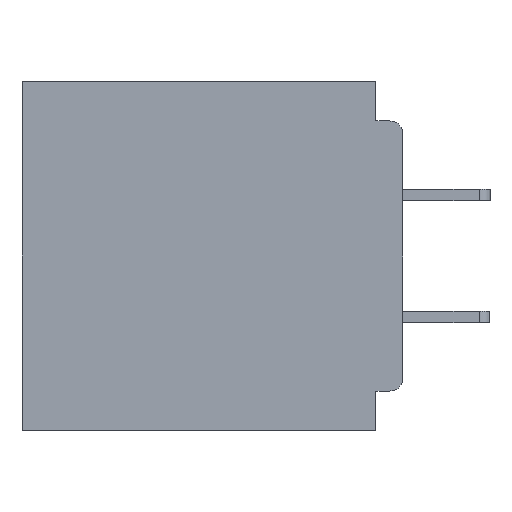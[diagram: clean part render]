
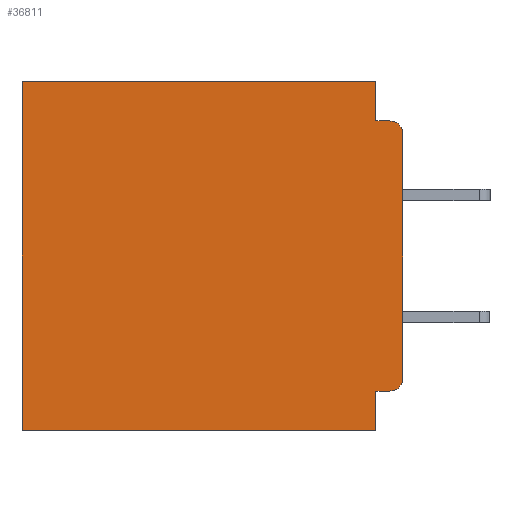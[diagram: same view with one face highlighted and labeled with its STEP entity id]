
A CAD part, left-side view. The second image highlights one B-rep face of the part: STEP entity #36811.
In plain terms, the highlighted planar face has unit normal (-1, 0, 0).
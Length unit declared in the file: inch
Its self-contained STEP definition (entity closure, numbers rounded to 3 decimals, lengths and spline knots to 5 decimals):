
#180 = LINE ( 'NONE', #29104, #8390 ) ;
#1345 = VERTEX_POINT ( 'NONE', #10909 ) ;
#2168 = DIRECTION ( 'NONE',  ( -1., 0., 0. ) ) ;
#2389 = CARTESIAN_POINT ( 'NONE',  ( 0.3, 0., -0.355 ) ) ;
#2405 = CARTESIAN_POINT ( 'NONE',  ( 0.3, 0., -0.34 ) ) ;
#3158 = CARTESIAN_POINT ( 'NONE',  ( 0.3, 0., -0.4 ) ) ;
#3338 = LINE ( 'NONE', #4510, #16851 ) ;
#3372 = CARTESIAN_POINT ( 'NONE',  ( 0.3, 0.015, -0.06 ) ) ;
#4238 = LINE ( 'NONE', #2389, #20634 ) ;
#4364 = VECTOR ( 'NONE', #32236, 39.37008 ) ;
#4455 = AXIS2_PLACEMENT_3D ( 'NONE', #7632, #10760, #32193 ) ;
#4510 = CARTESIAN_POINT ( 'NONE',  ( 0.3, 0., 0. ) ) ;
#4531 = PLANE ( 'NONE',  #4455 ) ;
#4718 = VERTEX_POINT ( 'NONE', #17786 ) ;
#5389 = CARTESIAN_POINT ( 'NONE',  ( 0.3, 0.031, -0.045 ) ) ;
#5960 = VERTEX_POINT ( 'NONE', #30890 ) ;
#6119 = VECTOR ( 'NONE', #23405, 39.37008 ) ;
#6398 = CARTESIAN_POINT ( 'NONE',  ( 0.3, 0.031, -0.355 ) ) ;
#6465 = DIRECTION ( 'NONE',  ( 0., 0., -1. ) ) ;
#7095 = LINE ( 'NONE', #20351, #6119 ) ;
#7237 = VECTOR ( 'NONE', #30842, 39.37008 ) ;
#7554 = VERTEX_POINT ( 'NONE', #36003 ) ;
#7614 = DIRECTION ( 'NONE',  ( 0., 1., 0. ) ) ;
#7632 = CARTESIAN_POINT ( 'NONE',  ( 0.3, 0., -0.4 ) ) ;
#7782 = EDGE_LOOP ( 'NONE', ( #23162, #24529, #25824, #27682, #28188, #29527, #30024, #30924, #31496, #32269 ) ) ;
#7936 = LINE ( 'NONE', #35241, #31489 ) ;
#8390 = VECTOR ( 'NONE', #16808, 39.37008 ) ;
#8595 = EDGE_CURVE ( 'NONE', #29781, #26532, #3338, .T. ) ;
#10760 = DIRECTION ( 'NONE',  ( 1., 0., 0. ) ) ;
#10909 = CARTESIAN_POINT ( 'NONE',  ( 0.3, 0.015, -0.045 ) ) ;
#13442 = EDGE_CURVE ( 'NONE', #5960, #7554, #7936, .T. ) ;
#13830 = CARTESIAN_POINT ( 'NONE',  ( 0.3, 0.437, 0. ) ) ;
#13949 = LINE ( 'NONE', #29820, #29267 ) ;
#14097 = VERTEX_POINT ( 'NONE', #5389 ) ;
#14298 = EDGE_CURVE ( 'NONE', #4718, #1345, #24211, .T. ) ;
#16808 = DIRECTION ( 'NONE',  ( 0., -1., 0. ) ) ;
#16851 = VECTOR ( 'NONE', #7614, 39.37008 ) ;
#16928 = DIRECTION ( 'NONE',  ( 0., 1., 0. ) ) ;
#17786 = CARTESIAN_POINT ( 'NONE',  ( 0.3, 0., -0.06 ) ) ;
#17795 = DIRECTION ( 'NONE',  ( 0., 1., 0. ) ) ;
#19812 = EDGE_CURVE ( 'NONE', #20315, #37203, #4238, .T. ) ;
#20315 = VERTEX_POINT ( 'NONE', #38423 ) ;
#20351 = CARTESIAN_POINT ( 'NONE',  ( 0.3, 0.031, 0. ) ) ;
#20634 = VECTOR ( 'NONE', #17795, 39.37008 ) ;
#20643 = CARTESIAN_POINT ( 'NONE',  ( 0.3, 0.015, -0.34 ) ) ;
#21900 = EDGE_CURVE ( 'NONE', #14097, #1345, #180, .T. ) ;
#23162 = ORIENTED_EDGE ( 'NONE', *, *, #24052, .F. ) ;
#23405 = DIRECTION ( 'NONE',  ( 0., 0., -1. ) ) ;
#23693 = DIRECTION ( 'NONE',  ( 0., 0., -1. ) ) ;
#24052 = EDGE_CURVE ( 'NONE', #4718, #35542, #31728, .T. ) ;
#24075 = CARTESIAN_POINT ( 'NONE',  ( 0.3, 0.031, 0. ) ) ;
#24211 = CIRCLE ( 'NONE', #37267, 0.015 ) ;
#24529 = ORIENTED_EDGE ( 'NONE', *, *, #14298, .T. ) ;
#24862 = DIRECTION ( 'NONE',  ( -1., 0., 0. ) ) ;
#25824 = ORIENTED_EDGE ( 'NONE', *, *, #21900, .F. ) ;
#26532 = VERTEX_POINT ( 'NONE', #13830 ) ;
#27682 = ORIENTED_EDGE ( 'NONE', *, *, #38051, .F. ) ;
#27984 = CIRCLE ( 'NONE', #35754, 0.015 ) ;
#28188 = ORIENTED_EDGE ( 'NONE', *, *, #8595, .T. ) ;
#29033 = CARTESIAN_POINT ( 'NONE',  ( 0.3, 0.031, -0.4 ) ) ;
#29104 = CARTESIAN_POINT ( 'NONE',  ( 0.3, 0., -0.045 ) ) ;
#29267 = VECTOR ( 'NONE', #35996, 39.37008 ) ;
#29527 = ORIENTED_EDGE ( 'NONE', *, *, #36347, .T. ) ;
#29781 = VERTEX_POINT ( 'NONE', #24075 ) ;
#29820 = CARTESIAN_POINT ( 'NONE',  ( 0.3, 0.437, -0.4 ) ) ;
#30024 = ORIENTED_EDGE ( 'NONE', *, *, #13442, .F. ) ;
#30842 = DIRECTION ( 'NONE',  ( 0., 0., -1. ) ) ;
#30890 = CARTESIAN_POINT ( 'NONE',  ( 0.3, 0.031, -0.4 ) ) ;
#30924 = ORIENTED_EDGE ( 'NONE', *, *, #35329, .F. ) ;
#31489 = VECTOR ( 'NONE', #16928, 39.37008 ) ;
#31496 = ORIENTED_EDGE ( 'NONE', *, *, #19812, .F. ) ;
#31728 = LINE ( 'NONE', #3158, #7237 ) ;
#32193 = DIRECTION ( 'NONE',  ( 0., 0., -1. ) ) ;
#32236 = DIRECTION ( 'NONE',  ( 0., 0., -1. ) ) ;
#32269 = ORIENTED_EDGE ( 'NONE', *, *, #33003, .T. ) ;
#33003 = EDGE_CURVE ( 'NONE', #20315, #35542, #27984, .T. ) ;
#35241 = CARTESIAN_POINT ( 'NONE',  ( 0.3, 0., -0.4 ) ) ;
#35329 = EDGE_CURVE ( 'NONE', #37203, #5960, #36079, .T. ) ;
#35542 = VERTEX_POINT ( 'NONE', #2405 ) ;
#35754 = AXIS2_PLACEMENT_3D ( 'NONE', #20643, #2168, #23693 ) ;
#35996 = DIRECTION ( 'NONE',  ( 0., 0., -1. ) ) ;
#36003 = CARTESIAN_POINT ( 'NONE',  ( 0.3, 0.437, -0.4 ) ) ;
#36079 = LINE ( 'NONE', #29033, #4364 ) ;
#36347 = EDGE_CURVE ( 'NONE', #26532, #7554, #13949, .T. ) ;
#36811 = ADVANCED_FACE ( 'NONE', ( #38830 ), #4531, .F. ) ;
#37203 = VERTEX_POINT ( 'NONE', #6398 ) ;
#37267 = AXIS2_PLACEMENT_3D ( 'NONE', #3372, #24862, #6465 ) ;
#38051 = EDGE_CURVE ( 'NONE', #29781, #14097, #7095, .T. ) ;
#38423 = CARTESIAN_POINT ( 'NONE',  ( 0.3, 0.015, -0.355 ) ) ;
#38830 = FACE_OUTER_BOUND ( 'NONE', #7782, .T. ) ;
